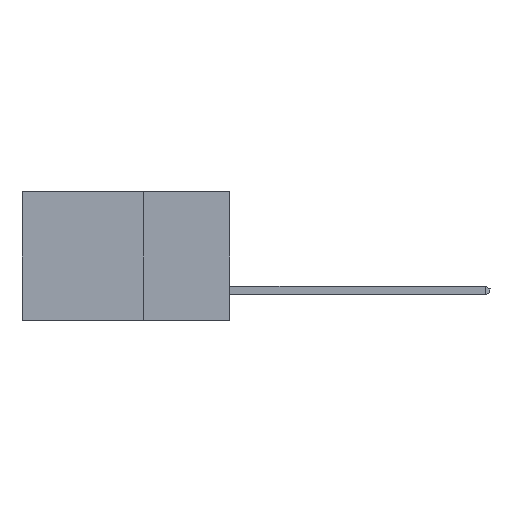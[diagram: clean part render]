
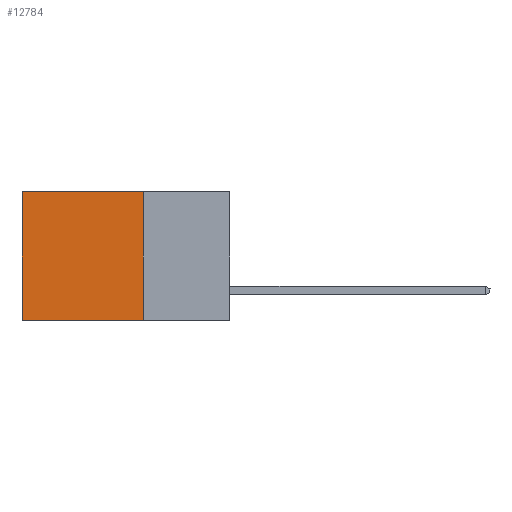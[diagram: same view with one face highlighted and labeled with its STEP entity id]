
A CAD part, left-side view. The second image highlights one B-rep face of the part: STEP entity #12784.
In plain terms, the highlighted planar face has unit normal (-1, 0, 0).
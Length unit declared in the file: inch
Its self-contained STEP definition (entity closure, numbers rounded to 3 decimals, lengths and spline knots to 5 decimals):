
#215 = CARTESIAN_POINT ( 'NONE',  ( 0.2615, 0.25, 0. ) ) ;
#783 = DIRECTION ( 'NONE',  ( 1., 0., 0. ) ) ;
#1719 = EDGE_LOOP ( 'NONE', ( #3050, #3542, #5975, #8722 ) ) ;
#1842 = VERTEX_POINT ( 'NONE', #9132 ) ;
#2341 = CARTESIAN_POINT ( 'NONE',  ( 0.2615, 0.25, 0. ) ) ;
#3050 = ORIENTED_EDGE ( 'NONE', *, *, #11375, .T. ) ;
#3191 = LINE ( 'NONE', #6209, #8126 ) ;
#3542 = ORIENTED_EDGE ( 'NONE', *, *, #6367, .F. ) ;
#4230 = DIRECTION ( 'NONE',  ( 0., 1., 0. ) ) ;
#4691 = VECTOR ( 'NONE', #4905, 39.37008 ) ;
#4905 = DIRECTION ( 'NONE',  ( 0., 1., 0. ) ) ;
#5882 = DIRECTION ( 'NONE',  ( 0., 0., -1. ) ) ;
#5975 = ORIENTED_EDGE ( 'NONE', *, *, #9882, .F. ) ;
#6010 = VECTOR ( 'NONE', #5882, 39.37008 ) ;
#6206 = LINE ( 'NONE', #215, #12504 ) ;
#6209 = CARTESIAN_POINT ( 'NONE',  ( 0.2615, 0.6, -0.37 ) ) ;
#6220 = CARTESIAN_POINT ( 'NONE',  ( 0.2615, 0.25, -0.37 ) ) ;
#6367 = EDGE_CURVE ( 'NONE', #9593, #11807, #10014, .T. ) ;
#6966 = DIRECTION ( 'NONE',  ( 0., 0., -1. ) ) ;
#8107 = CARTESIAN_POINT ( 'NONE',  ( 0.2615, 0.25, -0.37 ) ) ;
#8126 = VECTOR ( 'NONE', #10273, 39.37008 ) ;
#8722 = ORIENTED_EDGE ( 'NONE', *, *, #10059, .T. ) ;
#8807 = CARTESIAN_POINT ( 'NONE',  ( 0.2615, 0.25, -0.37 ) ) ;
#9132 = CARTESIAN_POINT ( 'NONE',  ( 0.2615, 0.6, 0. ) ) ;
#9593 = VERTEX_POINT ( 'NONE', #6220 ) ;
#9882 = EDGE_CURVE ( 'NONE', #11405, #9593, #12832, .T. ) ;
#9907 = CARTESIAN_POINT ( 'NONE',  ( 0.2615, 0.25, -0.37 ) ) ;
#10014 = LINE ( 'NONE', #8107, #4691 ) ;
#10059 = EDGE_CURVE ( 'NONE', #11405, #1842, #6206, .T. ) ;
#10189 = CARTESIAN_POINT ( 'NONE',  ( 0.2615, 0.6, -0.37 ) ) ;
#10273 = DIRECTION ( 'NONE',  ( 0., 0., -1. ) ) ;
#10773 = PLANE ( 'NONE',  #12320 ) ;
#11375 = EDGE_CURVE ( 'NONE', #1842, #11807, #3191, .T. ) ;
#11405 = VERTEX_POINT ( 'NONE', #2341 ) ;
#11807 = VERTEX_POINT ( 'NONE', #10189 ) ;
#11834 = FACE_OUTER_BOUND ( 'NONE', #1719, .T. ) ;
#12320 = AXIS2_PLACEMENT_3D ( 'NONE', #9907, #783, #6966 ) ;
#12504 = VECTOR ( 'NONE', #4230, 39.37008 ) ;
#12784 = ADVANCED_FACE ( 'NONE', ( #11834 ), #10773, .F. ) ;
#12832 = LINE ( 'NONE', #8807, #6010 ) ;
